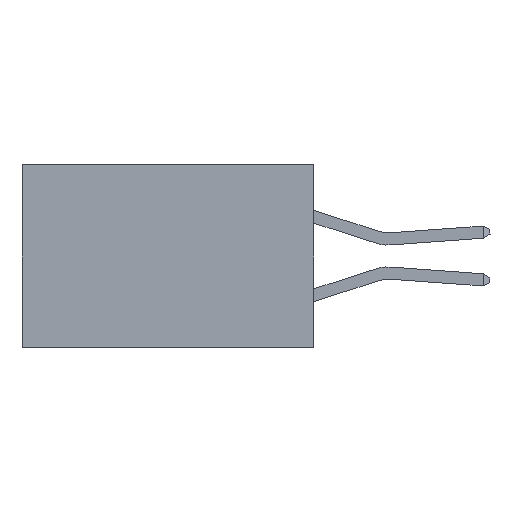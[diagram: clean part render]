
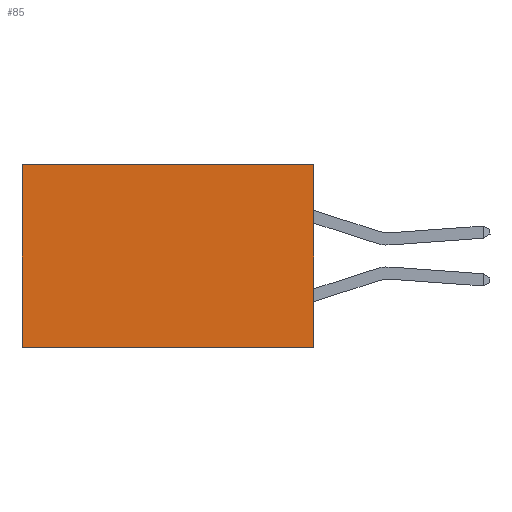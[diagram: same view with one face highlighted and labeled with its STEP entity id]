
A CAD part, left-side view. The second image highlights one B-rep face of the part: STEP entity #85.
In plain terms, the highlighted planar face has unit normal (-1, 0, 0).
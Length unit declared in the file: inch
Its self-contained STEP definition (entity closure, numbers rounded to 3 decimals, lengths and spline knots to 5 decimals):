
#59 = CARTESIAN_POINT ( 'NONE',  ( 0.2875, 0.6, 0. ) ) ;
#85 = ADVANCED_FACE ( 'NONE', ( #4131 ), #15270, .F. ) ;
#280 = EDGE_CURVE ( 'NONE', #318, #13663, #9594, .T. ) ;
#318 = VERTEX_POINT ( 'NONE', #7192 ) ;
#464 = VERTEX_POINT ( 'NONE', #12219 ) ;
#1001 = EDGE_CURVE ( 'NONE', #464, #318, #15389, .T. ) ;
#1080 = DIRECTION ( 'NONE',  ( 0., 0., -1. ) ) ;
#1943 = EDGE_LOOP ( 'NONE', ( #3878, #9776, #5850, #8610 ) ) ;
#2634 = VECTOR ( 'NONE', #10650, 39.37008 ) ;
#3343 = EDGE_CURVE ( 'NONE', #464, #7284, #4130, .T. ) ;
#3878 = ORIENTED_EDGE ( 'NONE', *, *, #12762, .T. ) ;
#4130 = LINE ( 'NONE', #11058, #14263 ) ;
#4131 = FACE_OUTER_BOUND ( 'NONE', #1943, .T. ) ;
#4390 = DIRECTION ( 'NONE',  ( 0., 0., -1. ) ) ;
#4723 = VECTOR ( 'NONE', #1080, 39.37008 ) ;
#5690 = LINE ( 'NONE', #7063, #4723 ) ;
#5850 = ORIENTED_EDGE ( 'NONE', *, *, #1001, .F. ) ;
#7063 = CARTESIAN_POINT ( 'NONE',  ( 0.2875, 0.6, -0.375 ) ) ;
#7192 = CARTESIAN_POINT ( 'NONE',  ( 0.2875, 0., -0.375 ) ) ;
#7284 = VERTEX_POINT ( 'NONE', #59 ) ;
#8029 = CARTESIAN_POINT ( 'NONE',  ( 0.2875, 0., -0.375 ) ) ;
#8610 = ORIENTED_EDGE ( 'NONE', *, *, #3343, .T. ) ;
#9465 = CARTESIAN_POINT ( 'NONE',  ( 0.2875, 0., -0.375 ) ) ;
#9594 = LINE ( 'NONE', #9465, #2634 ) ;
#9776 = ORIENTED_EDGE ( 'NONE', *, *, #280, .F. ) ;
#10650 = DIRECTION ( 'NONE',  ( 0., 1., 0. ) ) ;
#11058 = CARTESIAN_POINT ( 'NONE',  ( 0.2875, 0., 0. ) ) ;
#12004 = VECTOR ( 'NONE', #4390, 39.37008 ) ;
#12219 = CARTESIAN_POINT ( 'NONE',  ( 0.2875, 0., 0. ) ) ;
#12607 = AXIS2_PLACEMENT_3D ( 'NONE', #8029, #14180, #15377 ) ;
#12762 = EDGE_CURVE ( 'NONE', #7284, #13663, #5690, .T. ) ;
#13663 = VERTEX_POINT ( 'NONE', #15043 ) ;
#13931 = CARTESIAN_POINT ( 'NONE',  ( 0.2875, 0., -0.375 ) ) ;
#14180 = DIRECTION ( 'NONE',  ( 1., 0., 0. ) ) ;
#14263 = VECTOR ( 'NONE', #14693, 39.37008 ) ;
#14693 = DIRECTION ( 'NONE',  ( 0., 1., 0. ) ) ;
#15043 = CARTESIAN_POINT ( 'NONE',  ( 0.2875, 0.6, -0.375 ) ) ;
#15270 = PLANE ( 'NONE',  #12607 ) ;
#15377 = DIRECTION ( 'NONE',  ( 0., 0., -1. ) ) ;
#15389 = LINE ( 'NONE', #13931, #12004 ) ;
